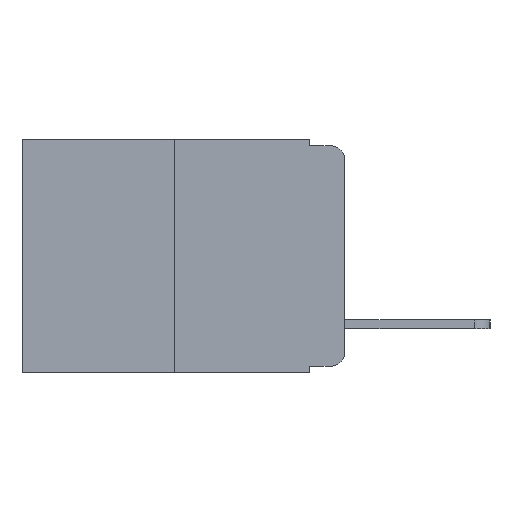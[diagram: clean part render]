
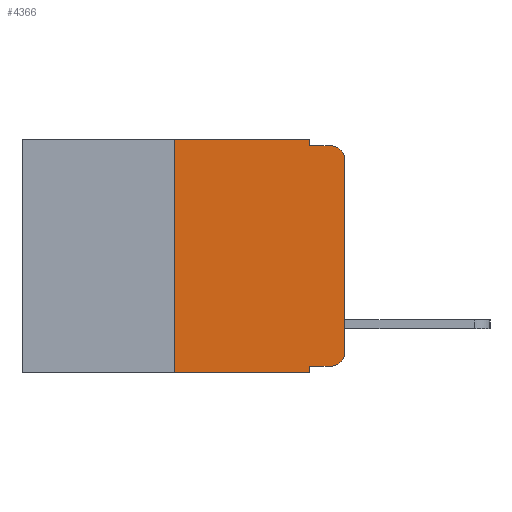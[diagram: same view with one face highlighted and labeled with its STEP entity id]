
A CAD part, left-side view. The second image highlights one B-rep face of the part: STEP entity #4366.
In plain terms, the highlighted planar face has unit normal (-1, 0, 0).
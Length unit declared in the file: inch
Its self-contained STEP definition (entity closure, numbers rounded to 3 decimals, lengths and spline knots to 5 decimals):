
#136 = VECTOR ( 'NONE', #16293, 39.37008 ) ;
#1169 = VERTEX_POINT ( 'NONE', #3108 ) ;
#1229 = EDGE_LOOP ( 'NONE', ( #3325, #5088, #2679, #2363, #9549, #3487, #2777, #8912, #7103, #6946 ) ) ;
#1292 = VERTEX_POINT ( 'NONE', #11667 ) ;
#1490 = CIRCLE ( 'NONE', #9641, 0.02 ) ;
#1795 = DIRECTION ( 'NONE',  ( 0., -1., 0. ) ) ;
#2363 = ORIENTED_EDGE ( 'NONE', *, *, #15874, .F. ) ;
#2679 = ORIENTED_EDGE ( 'NONE', *, *, #15870, .F. ) ;
#2777 = ORIENTED_EDGE ( 'NONE', *, *, #13951, .T. ) ;
#2953 = EDGE_CURVE ( 'NONE', #13492, #9440, #5045, .T. ) ;
#3108 = CARTESIAN_POINT ( 'NONE',  ( 0., 0.02, -0.01 ) ) ;
#3138 = DIRECTION ( 'NONE',  ( 0., -1., 0. ) ) ;
#3325 = ORIENTED_EDGE ( 'NONE', *, *, #15843, .T. ) ;
#3487 = ORIENTED_EDGE ( 'NONE', *, *, #17020, .F. ) ;
#3496 = LINE ( 'NONE', #5975, #17139 ) ;
#3501 = LINE ( 'NONE', #15518, #10714 ) ;
#3993 = CARTESIAN_POINT ( 'NONE',  ( 0., 0.051, 0. ) ) ;
#4366 = ADVANCED_FACE ( 'NONE', ( #13394 ), #16315, .F. ) ;
#4491 = CARTESIAN_POINT ( 'NONE',  ( 0., 0.473, 0. ) ) ;
#4631 = CARTESIAN_POINT ( 'NONE',  ( 0., 0.02, -0.03 ) ) ;
#4640 = DIRECTION ( 'NONE',  ( -1., 0., 0. ) ) ;
#5045 = LINE ( 'NONE', #4491, #136 ) ;
#5088 = ORIENTED_EDGE ( 'NONE', *, *, #15844, .T. ) ;
#5601 = EDGE_CURVE ( 'NONE', #9733, #14038, #3496, .T. ) ;
#5975 = CARTESIAN_POINT ( 'NONE',  ( 0., 0.051, -0.333 ) ) ;
#6133 = DIRECTION ( 'NONE',  ( 0., 0., 1. ) ) ;
#6207 = DIRECTION ( 'NONE',  ( 0., 0., -1. ) ) ;
#6569 = CARTESIAN_POINT ( 'NONE',  ( 0., 0.25, 0. ) ) ;
#6946 = ORIENTED_EDGE ( 'NONE', *, *, #7514, .T. ) ;
#6994 = AXIS2_PLACEMENT_3D ( 'NONE', #4631, #14255, #6207 ) ;
#7103 = ORIENTED_EDGE ( 'NONE', *, *, #5601, .T. ) ;
#7422 = VECTOR ( 'NONE', #1795, 39.37008 ) ;
#7514 = EDGE_CURVE ( 'NONE', #14038, #1292, #1490, .T. ) ;
#7596 = VERTEX_POINT ( 'NONE', #7725 ) ;
#7725 = CARTESIAN_POINT ( 'NONE',  ( 0., 0., -0.03 ) ) ;
#7962 = LINE ( 'NONE', #10385, #17513 ) ;
#8912 = ORIENTED_EDGE ( 'NONE', *, *, #15887, .F. ) ;
#9048 = CARTESIAN_POINT ( 'NONE',  ( 0., 0.051, -0.343 ) ) ;
#9417 = VERTEX_POINT ( 'NONE', #13652 ) ;
#9440 = VERTEX_POINT ( 'NONE', #3993 ) ;
#9549 = ORIENTED_EDGE ( 'NONE', *, *, #2953, .F. ) ;
#9551 = VERTEX_POINT ( 'NONE', #17736 ) ;
#9641 = AXIS2_PLACEMENT_3D ( 'NONE', #13015, #4640, #14263 ) ;
#9733 = VERTEX_POINT ( 'NONE', #11692 ) ;
#9911 = DIRECTION ( 'NONE',  ( 0., 0., -1. ) ) ;
#10181 = DIRECTION ( 'NONE',  ( 0., -1., 0. ) ) ;
#10385 = CARTESIAN_POINT ( 'NONE',  ( 0., 0.051, 0. ) ) ;
#10589 = VERTEX_POINT ( 'NONE', #9048 ) ;
#10714 = VECTOR ( 'NONE', #3138, 39.37008 ) ;
#10724 = DIRECTION ( 'NONE',  ( 0., 0., 1. ) ) ;
#11019 = LINE ( 'NONE', #11973, #7422 ) ;
#11132 = CIRCLE ( 'NONE', #6994, 0.02 ) ;
#11546 = LINE ( 'NONE', #16752, #14557 ) ;
#11667 = CARTESIAN_POINT ( 'NONE',  ( 0., 0., -0.313 ) ) ;
#11692 = CARTESIAN_POINT ( 'NONE',  ( 0., 0.051, -0.333 ) ) ;
#11973 = CARTESIAN_POINT ( 'NONE',  ( 0., 0.473, -0.343 ) ) ;
#12576 = CARTESIAN_POINT ( 'NONE',  ( 0., 0.25, 0. ) ) ;
#13015 = CARTESIAN_POINT ( 'NONE',  ( 0., 0.02, -0.313 ) ) ;
#13069 = CARTESIAN_POINT ( 'NONE',  ( 0., 0.051, 0. ) ) ;
#13394 = FACE_OUTER_BOUND ( 'NONE', #1229, .T. ) ;
#13492 = VERTEX_POINT ( 'NONE', #12576 ) ;
#13577 = VECTOR ( 'NONE', #10724, 39.37008 ) ;
#13652 = CARTESIAN_POINT ( 'NONE',  ( 0., 0.051, -0.01 ) ) ;
#13791 = VECTOR ( 'NONE', #16858, 39.37008 ) ;
#13913 = AXIS2_PLACEMENT_3D ( 'NONE', #15087, #17620, #9911 ) ;
#13951 = EDGE_CURVE ( 'NONE', #9551, #10589, #11019, .T. ) ;
#14038 = VERTEX_POINT ( 'NONE', #17255 ) ;
#14255 = DIRECTION ( 'NONE',  ( -1., 0., 0. ) ) ;
#14263 = DIRECTION ( 'NONE',  ( 0., 0., -1. ) ) ;
#14311 = DIRECTION ( 'NONE',  ( 0., 0., -1. ) ) ;
#14557 = VECTOR ( 'NONE', #6133, 39.37008 ) ;
#15087 = CARTESIAN_POINT ( 'NONE',  ( 0., 0.473, 0. ) ) ;
#15518 = CARTESIAN_POINT ( 'NONE',  ( 0., 0.051, -0.01 ) ) ;
#15843 = EDGE_CURVE ( 'NONE', #1292, #7596, #11546, .T. ) ;
#15844 = EDGE_CURVE ( 'NONE', #7596, #1169, #11132, .T. ) ;
#15870 = EDGE_CURVE ( 'NONE', #9417, #1169, #3501, .T. ) ;
#15874 = EDGE_CURVE ( 'NONE', #9440, #9417, #7962, .T. ) ;
#15887 = EDGE_CURVE ( 'NONE', #9733, #10589, #17143, .T. ) ;
#16293 = DIRECTION ( 'NONE',  ( 0., -1., 0. ) ) ;
#16315 = PLANE ( 'NONE',  #13913 ) ;
#16752 = CARTESIAN_POINT ( 'NONE',  ( 0., 0., 0. ) ) ;
#16858 = DIRECTION ( 'NONE',  ( 0., 0., -1. ) ) ;
#16909 = LINE ( 'NONE', #6569, #13577 ) ;
#17020 = EDGE_CURVE ( 'NONE', #9551, #13492, #16909, .T. ) ;
#17139 = VECTOR ( 'NONE', #10181, 39.37008 ) ;
#17143 = LINE ( 'NONE', #13069, #13791 ) ;
#17255 = CARTESIAN_POINT ( 'NONE',  ( 0., 0.02, -0.333 ) ) ;
#17513 = VECTOR ( 'NONE', #14311, 39.37008 ) ;
#17620 = DIRECTION ( 'NONE',  ( 1., 0., 0. ) ) ;
#17736 = CARTESIAN_POINT ( 'NONE',  ( 0., 0.25, -0.343 ) ) ;
